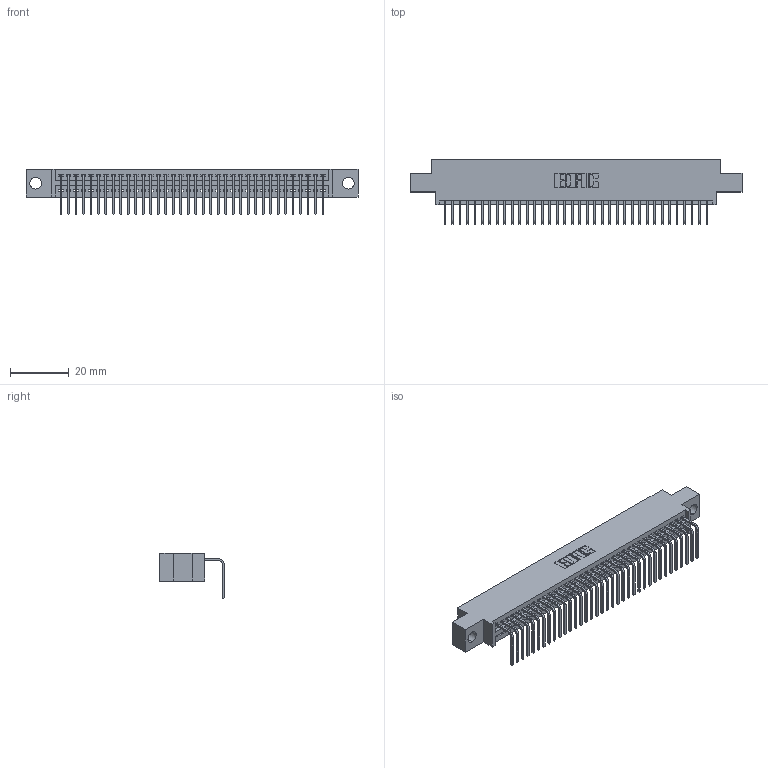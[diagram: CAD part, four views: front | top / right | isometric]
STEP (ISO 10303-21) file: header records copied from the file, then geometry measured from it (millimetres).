
FILE_DESCRIPTION (( 'STEP AP203' ), '1' );
FILE_NAME ('395-036-558-604.STEP', '2018-11-13T21:32:07', ( '' ), ( '' ), 'SwSTEP 2.0', 'SolidWorks 2016', '' );
FILE_SCHEMA (( 'CONFIG_CONTROL_DESIGN' ));
Length unit declared in the file: inch
Products named in the file (3): 345 Part_0.170 Offset - 0.156 Dia-TH; 345-292-001_558 Tail - 2; 395-036-558-604
Assembly tree (37 placements, depth 2):
  395-036-558-604
    345 Part_0.170 Offset - 0.156 Dia-TH
    345-292-001_558 Tail - 2  x36
Bounding box: 112.65 x 21.83 x 15.37 mm (x, y, z)
Volume: 10569.1 mm3; surface area: 14603.9 mm2
Topology: 37 solids, 37 shells, 2290 faces, 6905 edges, 4554 vertices
Faces by surface type: plane 1596, cylinder 694
Entity records: 28121 total; most frequent: CARTESIAN_POINT 4880, ORIENTED_EDGE 4850, DIRECTION 4269, EDGE_CURVE 2425, VECTOR 2149, LINE 2149, VERTEX_POINT 1614, AXIS2_PLACEMENT_3D 1060
